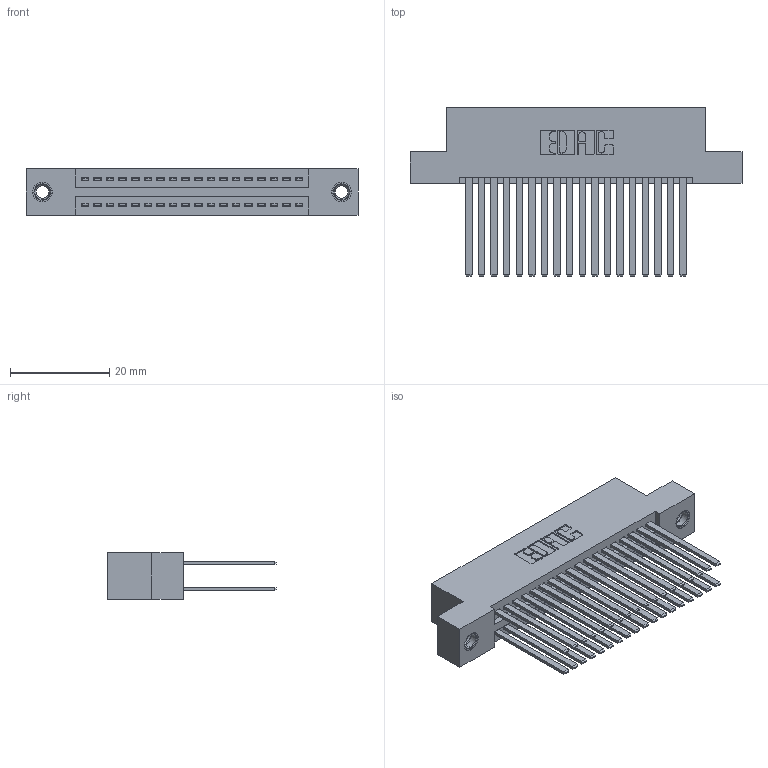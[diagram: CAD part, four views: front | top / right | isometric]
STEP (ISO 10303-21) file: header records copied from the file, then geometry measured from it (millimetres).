
FILE_DESCRIPTION (( 'STEP AP203' ), '1' );
FILE_NAME ('345-036-544-207.STEP', '2018-08-29T23:44:11', ( '' ), ( '' ), 'SwSTEP 2.0', 'SolidWorks 2016', '' );
FILE_SCHEMA (( 'CONFIG_CONTROL_DESIGN' ));
Length unit declared in the file: inch
Products named in the file (4): 345 Part_Flush Mounting Lugs - 0.156 Dia-TI; 345-292-001_345-293-144; 345-250-001_345-250-005-103; 345-036-544-207
Assembly tree (39 placements, depth 2):
  345-036-544-207
    345 Part_Flush Mounting Lugs - 0.156 Dia-TI
    345-292-001_345-293-144  x36
    345-250-001_345-250-005-103  x2
Bounding box: 66.93 x 33.96 x 9.4 mm (x, y, z)
Volume: 6769.9 mm3; surface area: 11049.2 mm2
Topology: 39 solids, 39 shells, 1770 faces, 5193 edges, 3406 vertices
Faces by surface type: plane 1156, cylinder 598, cone 12, torus 4
Entity records: 18356 total; most frequent: CARTESIAN_POINT 3079, ORIENTED_EDGE 3006, DIRECTION 2769, EDGE_CURVE 1503, VECTOR 1283, LINE 1283, VERTEX_POINT 996, AXIS2_PLACEMENT_3D 743
